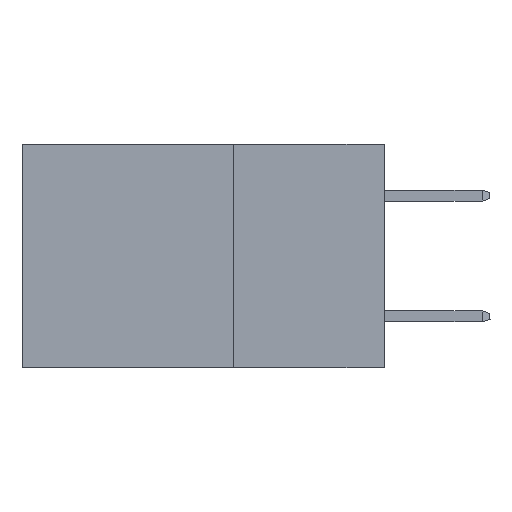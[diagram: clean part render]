
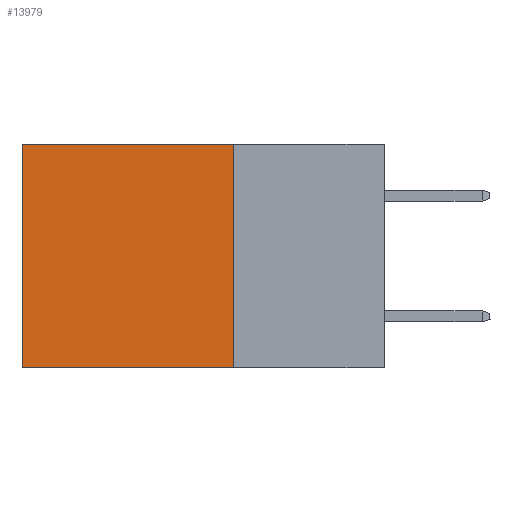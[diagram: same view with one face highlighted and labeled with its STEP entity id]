
A CAD part, left-side view. The second image highlights one B-rep face of the part: STEP entity #13979.
In plain terms, the highlighted planar face has unit normal (-1, 0, 0).
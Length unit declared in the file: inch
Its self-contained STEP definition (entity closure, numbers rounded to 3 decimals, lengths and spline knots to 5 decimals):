
#183 = VERTEX_POINT ( 'NONE', #5784 ) ;
#191 = VERTEX_POINT ( 'NONE', #7609 ) ;
#843 = LINE ( 'NONE', #18843, #16090 ) ;
#1717 = AXIS2_PLACEMENT_3D ( 'NONE', #4100, #5591, #15877 ) ;
#2376 = VERTEX_POINT ( 'NONE', #18705 ) ;
#2437 = VECTOR ( 'NONE', #15758, 39.37008 ) ;
#2783 = EDGE_LOOP ( 'NONE', ( #16535, #8003, #9566, #14461 ) ) ;
#3982 = CARTESIAN_POINT ( 'NONE',  ( 0.2615, 0.25, -0.37 ) ) ;
#4100 = CARTESIAN_POINT ( 'NONE',  ( 0.2615, 0.25, -0.37 ) ) ;
#4227 = VERTEX_POINT ( 'NONE', #10134 ) ;
#4476 = CARTESIAN_POINT ( 'NONE',  ( 0.2615, 0.6, -0.37 ) ) ;
#5545 = DIRECTION ( 'NONE',  ( 0., 0., -1. ) ) ;
#5591 = DIRECTION ( 'NONE',  ( 1., 0., 0. ) ) ;
#5784 = CARTESIAN_POINT ( 'NONE',  ( 0.2615, 0.25, -0.37 ) ) ;
#7438 = VECTOR ( 'NONE', #5545, 39.37008 ) ;
#7479 = VECTOR ( 'NONE', #16256, 39.37008 ) ;
#7609 = CARTESIAN_POINT ( 'NONE',  ( 0.2615, 0.6, 0. ) ) ;
#7958 = LINE ( 'NONE', #4476, #7479 ) ;
#8003 = ORIENTED_EDGE ( 'NONE', *, *, #9528, .F. ) ;
#8933 = EDGE_CURVE ( 'NONE', #4227, #191, #843, .T. ) ;
#9528 = EDGE_CURVE ( 'NONE', #183, #2376, #18077, .T. ) ;
#9566 = ORIENTED_EDGE ( 'NONE', *, *, #12208, .F. ) ;
#10134 = CARTESIAN_POINT ( 'NONE',  ( 0.2615, 0.25, 0. ) ) ;
#12208 = EDGE_CURVE ( 'NONE', #4227, #183, #18634, .T. ) ;
#13979 = ADVANCED_FACE ( 'NONE', ( #15457 ), #14307, .F. ) ;
#14307 = PLANE ( 'NONE',  #1717 ) ;
#14461 = ORIENTED_EDGE ( 'NONE', *, *, #8933, .T. ) ;
#15457 = FACE_OUTER_BOUND ( 'NONE', #2783, .T. ) ;
#15758 = DIRECTION ( 'NONE',  ( 0., 1., 0. ) ) ;
#15877 = DIRECTION ( 'NONE',  ( 0., 0., -1. ) ) ;
#15962 = DIRECTION ( 'NONE',  ( 0., 1., 0. ) ) ;
#16090 = VECTOR ( 'NONE', #15962, 39.37008 ) ;
#16256 = DIRECTION ( 'NONE',  ( 0., 0., -1. ) ) ;
#16535 = ORIENTED_EDGE ( 'NONE', *, *, #16904, .T. ) ;
#16904 = EDGE_CURVE ( 'NONE', #191, #2376, #7958, .T. ) ;
#17279 = CARTESIAN_POINT ( 'NONE',  ( 0.2615, 0.25, -0.37 ) ) ;
#18077 = LINE ( 'NONE', #3982, #2437 ) ;
#18634 = LINE ( 'NONE', #17279, #7438 ) ;
#18705 = CARTESIAN_POINT ( 'NONE',  ( 0.2615, 0.6, -0.37 ) ) ;
#18843 = CARTESIAN_POINT ( 'NONE',  ( 0.2615, 0.25, 0. ) ) ;
